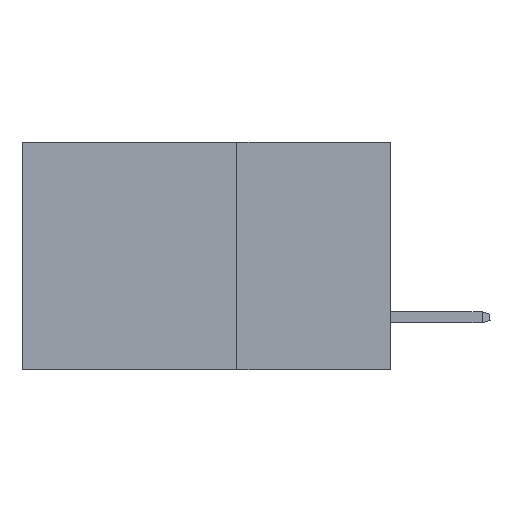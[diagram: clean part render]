
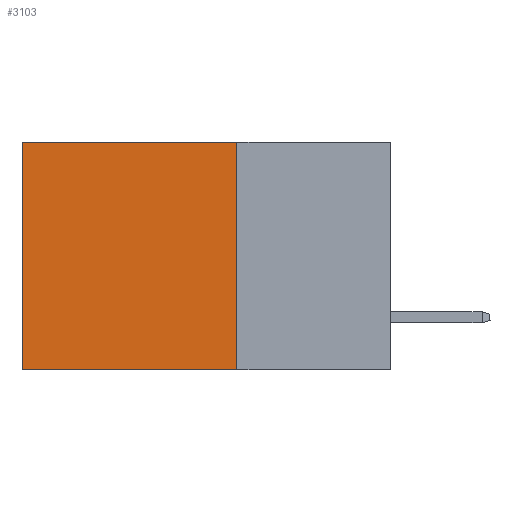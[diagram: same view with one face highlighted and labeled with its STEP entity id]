
A CAD part, left-side view. The second image highlights one B-rep face of the part: STEP entity #3103.
In plain terms, the highlighted planar face has unit normal (-1, 0, 0).
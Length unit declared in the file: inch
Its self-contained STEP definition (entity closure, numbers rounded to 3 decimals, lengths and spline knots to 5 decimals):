
#308 = VECTOR ( 'NONE', #7328, 39.37008 ) ;
#400 = VECTOR ( 'NONE', #7235, 39.37008 ) ;
#1993 = VERTEX_POINT ( 'NONE', #3481 ) ;
#2229 = CARTESIAN_POINT ( 'NONE',  ( 0.2875, 0.25, 0. ) ) ;
#3103 = ADVANCED_FACE ( 'NONE', ( #14462 ), #10651, .F. ) ;
#3168 = VERTEX_POINT ( 'NONE', #6047 ) ;
#3367 = EDGE_CURVE ( 'NONE', #12556, #3168, #13324, .T. ) ;
#3481 = CARTESIAN_POINT ( 'NONE',  ( 0.2875, 0.6, -0.37 ) ) ;
#3830 = AXIS2_PLACEMENT_3D ( 'NONE', #2229, #9521, #4639 ) ;
#4639 = DIRECTION ( 'NONE',  ( 0., 0., -1. ) ) ;
#5188 = EDGE_CURVE ( 'NONE', #13519, #1993, #11345, .T. ) ;
#5851 = VECTOR ( 'NONE', #9451, 39.37008 ) ;
#6047 = CARTESIAN_POINT ( 'NONE',  ( 0.2875, 0.6, 0. ) ) ;
#6088 = CARTESIAN_POINT ( 'NONE',  ( 0.2875, 0.25, 0. ) ) ;
#6881 = EDGE_CURVE ( 'NONE', #12556, #13519, #10372, .T. ) ;
#7035 = CARTESIAN_POINT ( 'NONE',  ( 0.2875, 0.6, 0. ) ) ;
#7235 = DIRECTION ( 'NONE',  ( 0., 0., -1. ) ) ;
#7328 = DIRECTION ( 'NONE',  ( 0., 1., 0. ) ) ;
#7356 = EDGE_CURVE ( 'NONE', #3168, #1993, #12065, .T. ) ;
#8849 = VECTOR ( 'NONE', #11889, 39.37008 ) ;
#9451 = DIRECTION ( 'NONE',  ( 0., 1., 0. ) ) ;
#9521 = DIRECTION ( 'NONE',  ( 1., 0., 0. ) ) ;
#10372 = LINE ( 'NONE', #6088, #400 ) ;
#10458 = CARTESIAN_POINT ( 'NONE',  ( 0.2875, 0.25, -0.37 ) ) ;
#10536 = EDGE_LOOP ( 'NONE', ( #11633, #11479, #12365, #13602 ) ) ;
#10651 = PLANE ( 'NONE',  #3830 ) ;
#11345 = LINE ( 'NONE', #13087, #5851 ) ;
#11479 = ORIENTED_EDGE ( 'NONE', *, *, #5188, .F. ) ;
#11633 = ORIENTED_EDGE ( 'NONE', *, *, #7356, .T. ) ;
#11853 = CARTESIAN_POINT ( 'NONE',  ( 0.2875, 0.25, 0. ) ) ;
#11889 = DIRECTION ( 'NONE',  ( 0., 0., -1. ) ) ;
#12065 = LINE ( 'NONE', #7035, #8849 ) ;
#12365 = ORIENTED_EDGE ( 'NONE', *, *, #6881, .F. ) ;
#12556 = VERTEX_POINT ( 'NONE', #11853 ) ;
#13087 = CARTESIAN_POINT ( 'NONE',  ( 0.2875, 0.25, -0.37 ) ) ;
#13324 = LINE ( 'NONE', #14661, #308 ) ;
#13519 = VERTEX_POINT ( 'NONE', #10458 ) ;
#13602 = ORIENTED_EDGE ( 'NONE', *, *, #3367, .T. ) ;
#14462 = FACE_OUTER_BOUND ( 'NONE', #10536, .T. ) ;
#14661 = CARTESIAN_POINT ( 'NONE',  ( 0.2875, 0.25, 0. ) ) ;
